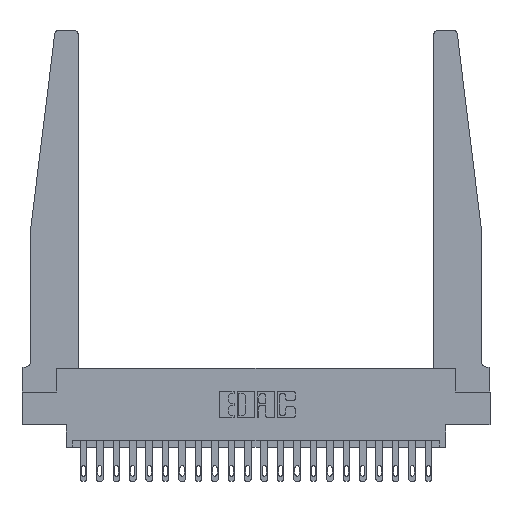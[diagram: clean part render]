
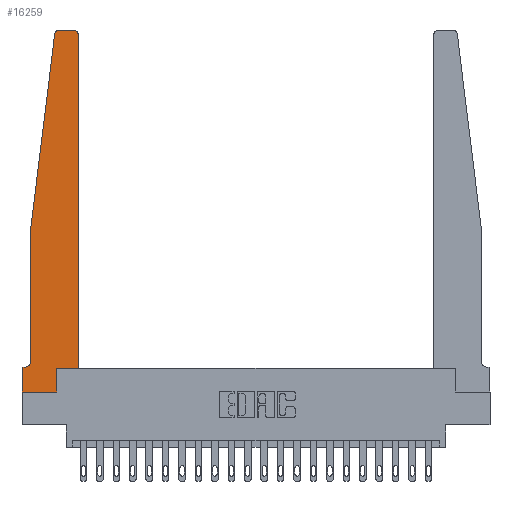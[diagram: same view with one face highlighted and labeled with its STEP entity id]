
A CAD part, top view. The second image highlights one B-rep face of the part: STEP entity #16259.
In plain terms, the highlighted planar face has unit normal (0, 0, 1).
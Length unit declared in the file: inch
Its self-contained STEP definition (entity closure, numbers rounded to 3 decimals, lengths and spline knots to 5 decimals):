
#68 = CARTESIAN_POINT ( 'NONE',  ( 0.395, 2.72, 0.37 ) ) ;
#94 = LINE ( 'NONE', #13866, #21001 ) ;
#113 = CARTESIAN_POINT ( 'NONE',  ( 0.425, 0.18, 0.37 ) ) ;
#294 = DIRECTION ( 'NONE',  ( 0., 0., 1. ) ) ;
#412 = DIRECTION ( 'NONE',  ( 0., 0., 1. ) ) ;
#624 = EDGE_CURVE ( 'NONE', #14099, #15210, #712, .T. ) ;
#711 = LINE ( 'NONE', #2416, #21167 ) ;
#712 = LINE ( 'NONE', #14465, #11826 ) ;
#759 = FACE_OUTER_BOUND ( 'NONE', #10394, .T. ) ;
#1097 = LINE ( 'NONE', #7966, #10820 ) ;
#1113 = CARTESIAN_POINT ( 'NONE',  ( 0.25, 2.75, 0.37 ) ) ;
#1528 = CARTESIAN_POINT ( 'NONE',  ( 0.2605, 0., 0.37 ) ) ;
#2221 = VECTOR ( 'NONE', #4988, 39.37008 ) ;
#2416 = CARTESIAN_POINT ( 'NONE',  ( 0.065, 0.1875, 0.37 ) ) ;
#2535 = CARTESIAN_POINT ( 'NONE',  ( 0.27653, 2.75, 0.37 ) ) ;
#2665 = VERTEX_POINT ( 'NONE', #11975 ) ;
#2877 = AXIS2_PLACEMENT_3D ( 'NONE', #7106, #12938, #14620 ) ;
#2945 = VERTEX_POINT ( 'NONE', #3555 ) ;
#3081 = VERTEX_POINT ( 'NONE', #2535 ) ;
#3555 = CARTESIAN_POINT ( 'NONE',  ( 0.015, 0.1875, 0.37 ) ) ;
#3974 = VECTOR ( 'NONE', #16544, 39.37008 ) ;
#4003 = CARTESIAN_POINT ( 'NONE',  ( 0.2605, 0.18, 0.37 ) ) ;
#4375 = VECTOR ( 'NONE', #4696, 39.37008 ) ;
#4696 = DIRECTION ( 'NONE',  ( -0.122, -0.992, 0. ) ) ;
#4905 = VERTEX_POINT ( 'NONE', #18182 ) ;
#4988 = DIRECTION ( 'NONE',  ( 0., 1., 0. ) ) ;
#5023 = EDGE_CURVE ( 'NONE', #2665, #3081, #9919, .T. ) ;
#5142 = EDGE_CURVE ( 'NONE', #3081, #5673, #9371, .T. ) ;
#5371 = DIRECTION ( 'NONE',  ( -1., 0., 0. ) ) ;
#5400 = AXIS2_PLACEMENT_3D ( 'NONE', #15881, #294, #8880 ) ;
#5673 = VERTEX_POINT ( 'NONE', #12026 ) ;
#5861 = DIRECTION ( 'NONE',  ( 1., 0., 0. ) ) ;
#6519 = CARTESIAN_POINT ( 'NONE',  ( 0.065, 0.2375, 0.37 ) ) ;
#7003 = LINE ( 'NONE', #113, #2221 ) ;
#7027 = VERTEX_POINT ( 'NONE', #4003 ) ;
#7106 = CARTESIAN_POINT ( 'NONE',  ( 0., 0.1875, 0.37 ) ) ;
#7531 = PLANE ( 'NONE',  #2877 ) ;
#7966 = CARTESIAN_POINT ( 'NONE',  ( 0.2605, 0.18, 0.37 ) ) ;
#8880 = DIRECTION ( 'NONE',  ( 1., 0., 0. ) ) ;
#9371 = CIRCLE ( 'NONE', #5400, 0.03 ) ;
#9376 = ORIENTED_EDGE ( 'NONE', *, *, #624, .T. ) ;
#9773 = LINE ( 'NONE', #14832, #4375 ) ;
#9919 = LINE ( 'NONE', #1113, #11888 ) ;
#10346 = DIRECTION ( 'NONE',  ( 0., 0., -1. ) ) ;
#10394 = EDGE_LOOP ( 'NONE', ( #13824, #14988, #18544, #9376, #12429, #19927, #14293, #20156, #10831, #17682, #18962, #13432 ) ) ;
#10820 = VECTOR ( 'NONE', #14846, 39.37008 ) ;
#10831 = ORIENTED_EDGE ( 'NONE', *, *, #16472, .T. ) ;
#11826 = VECTOR ( 'NONE', #14135, 39.37008 ) ;
#11888 = VECTOR ( 'NONE', #13397, 39.37008 ) ;
#11925 = CARTESIAN_POINT ( 'NONE',  ( 0.015, 0.2375, 0.37 ) ) ;
#11926 = EDGE_CURVE ( 'NONE', #2945, #15668, #711, .T. ) ;
#11975 = CARTESIAN_POINT ( 'NONE',  ( 0.395, 2.75, 0.37 ) ) ;
#12026 = CARTESIAN_POINT ( 'NONE',  ( 0.24675, 2.72367, 0.37 ) ) ;
#12272 = CARTESIAN_POINT ( 'NONE',  ( 0.065, 1.25, 0.37 ) ) ;
#12429 = ORIENTED_EDGE ( 'NONE', *, *, #16529, .T. ) ;
#12851 = EDGE_CURVE ( 'NONE', #7027, #16686, #14414, .T. ) ;
#12938 = DIRECTION ( 'NONE',  ( 0., 0., 1. ) ) ;
#13360 = LINE ( 'NONE', #13469, #3974 ) ;
#13397 = DIRECTION ( 'NONE',  ( -1., 0., 0. ) ) ;
#13432 = ORIENTED_EDGE ( 'NONE', *, *, #15261, .T. ) ;
#13469 = CARTESIAN_POINT ( 'NONE',  ( 0., 0., 0.37 ) ) ;
#13824 = ORIENTED_EDGE ( 'NONE', *, *, #5023, .T. ) ;
#13866 = CARTESIAN_POINT ( 'NONE',  ( 0., 0., 0.37 ) ) ;
#14099 = VERTEX_POINT ( 'NONE', #12272 ) ;
#14135 = DIRECTION ( 'NONE',  ( 0., -1., 0. ) ) ;
#14293 = ORIENTED_EDGE ( 'NONE', *, *, #16858, .T. ) ;
#14301 = CARTESIAN_POINT ( 'NONE',  ( 0.425, 0.18, 0.37 ) ) ;
#14414 = LINE ( 'NONE', #14301, #20801 ) ;
#14465 = CARTESIAN_POINT ( 'NONE',  ( 0.065, 1.25, 0.37 ) ) ;
#14620 = DIRECTION ( 'NONE',  ( 1., 0., 0. ) ) ;
#14832 = CARTESIAN_POINT ( 'NONE',  ( 0.065, 1.25, 0.37 ) ) ;
#14846 = DIRECTION ( 'NONE',  ( 0., 1., 0. ) ) ;
#14988 = ORIENTED_EDGE ( 'NONE', *, *, #5142, .T. ) ;
#15210 = VERTEX_POINT ( 'NONE', #6519 ) ;
#15261 = EDGE_CURVE ( 'NONE', #19872, #2665, #17974, .T. ) ;
#15668 = VERTEX_POINT ( 'NONE', #20263 ) ;
#15850 = CIRCLE ( 'NONE', #21631, 0.05 ) ;
#15881 = CARTESIAN_POINT ( 'NONE',  ( 0.27653, 2.72, 0.37 ) ) ;
#16128 = CARTESIAN_POINT ( 'NONE',  ( 0.425, 2.72, 0.37 ) ) ;
#16259 = ADVANCED_FACE ( 'NONE', ( #759 ), #7531, .T. ) ;
#16472 = EDGE_CURVE ( 'NONE', #21862, #7027, #1097, .T. ) ;
#16529 = EDGE_CURVE ( 'NONE', #15210, #2945, #15850, .T. ) ;
#16544 = DIRECTION ( 'NONE',  ( 0., -1., 0. ) ) ;
#16686 = VERTEX_POINT ( 'NONE', #18021 ) ;
#16858 = EDGE_CURVE ( 'NONE', #15668, #4905, #13360, .T. ) ;
#16881 = AXIS2_PLACEMENT_3D ( 'NONE', #68, #412, #21082 ) ;
#17682 = ORIENTED_EDGE ( 'NONE', *, *, #12851, .T. ) ;
#17974 = CIRCLE ( 'NONE', #16881, 0.03 ) ;
#18021 = CARTESIAN_POINT ( 'NONE',  ( 0.425, 0.18, 0.37 ) ) ;
#18182 = CARTESIAN_POINT ( 'NONE',  ( 0., 0., 0.37 ) ) ;
#18544 = ORIENTED_EDGE ( 'NONE', *, *, #20524, .T. ) ;
#18765 = EDGE_CURVE ( 'NONE', #16686, #19872, #7003, .T. ) ;
#18962 = ORIENTED_EDGE ( 'NONE', *, *, #18765, .T. ) ;
#19822 = EDGE_CURVE ( 'NONE', #4905, #21862, #94, .T. ) ;
#19872 = VERTEX_POINT ( 'NONE', #16128 ) ;
#19912 = DIRECTION ( 'NONE',  ( -1., 0., 0. ) ) ;
#19927 = ORIENTED_EDGE ( 'NONE', *, *, #11926, .T. ) ;
#20156 = ORIENTED_EDGE ( 'NONE', *, *, #19822, .T. ) ;
#20263 = CARTESIAN_POINT ( 'NONE',  ( 0., 0.1875, 0.37 ) ) ;
#20524 = EDGE_CURVE ( 'NONE', #5673, #14099, #9773, .T. ) ;
#20782 = DIRECTION ( 'NONE',  ( 1., 0., 0. ) ) ;
#20801 = VECTOR ( 'NONE', #5861, 39.37008 ) ;
#21001 = VECTOR ( 'NONE', #20782, 39.37008 ) ;
#21082 = DIRECTION ( 'NONE',  ( 1., 0., 0. ) ) ;
#21167 = VECTOR ( 'NONE', #19912, 39.37008 ) ;
#21631 = AXIS2_PLACEMENT_3D ( 'NONE', #11925, #10346, #5371 ) ;
#21862 = VERTEX_POINT ( 'NONE', #1528 ) ;
